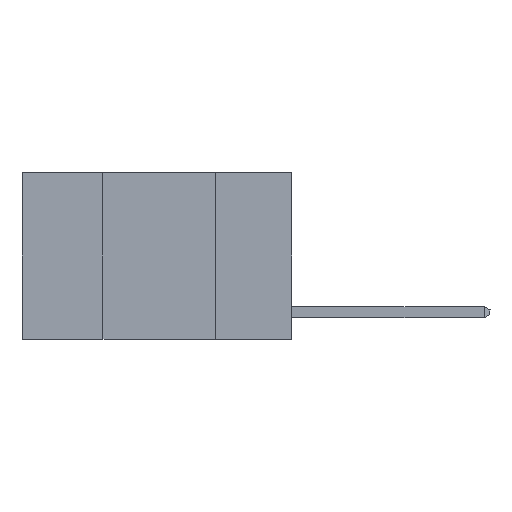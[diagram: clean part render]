
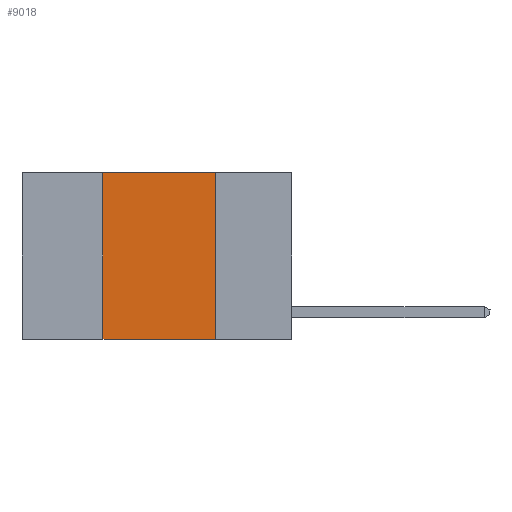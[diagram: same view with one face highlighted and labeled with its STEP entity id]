
A CAD part, left-side view. The second image highlights one B-rep face of the part: STEP entity #9018.
In plain terms, the highlighted planar face has unit normal (-1, 0, 0).
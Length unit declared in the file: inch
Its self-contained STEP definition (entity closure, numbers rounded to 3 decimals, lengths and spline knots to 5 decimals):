
#171 = VECTOR ( 'NONE', #7071, 39.37008 ) ;
#3466 = VERTEX_POINT ( 'NONE', #5015 ) ;
#3481 = CARTESIAN_POINT ( 'NONE',  ( 0., 0.6, -0.37 ) ) ;
#3925 = VECTOR ( 'NONE', #14369, 39.37008 ) ;
#5015 = CARTESIAN_POINT ( 'NONE',  ( 0., 0.17, 0. ) ) ;
#5437 = CARTESIAN_POINT ( 'NONE',  ( 0., 0.42, -0.37 ) ) ;
#6284 = DIRECTION ( 'NONE',  ( 1., 0., 0. ) ) ;
#7063 = VECTOR ( 'NONE', #12515, 39.37008 ) ;
#7071 = DIRECTION ( 'NONE',  ( 0., 0., 1. ) ) ;
#7338 = LINE ( 'NONE', #7885, #14939 ) ;
#7378 = ORIENTED_EDGE ( 'NONE', *, *, #17467, .F. ) ;
#7527 = AXIS2_PLACEMENT_3D ( 'NONE', #15374, #6284, #16900 ) ;
#7839 = VERTEX_POINT ( 'NONE', #8434 ) ;
#7885 = CARTESIAN_POINT ( 'NONE',  ( 0., 0.17, 0. ) ) ;
#7903 = EDGE_CURVE ( 'NONE', #10601, #18689, #12953, .T. ) ;
#8434 = CARTESIAN_POINT ( 'NONE',  ( 0., 0.17, -0.37 ) ) ;
#9018 = ADVANCED_FACE ( 'NONE', ( #11711 ), #16834, .F. ) ;
#9217 = EDGE_CURVE ( 'NONE', #18689, #3466, #11939, .T. ) ;
#9403 = DIRECTION ( 'NONE',  ( 0., 0., -1. ) ) ;
#10601 = VERTEX_POINT ( 'NONE', #5437 ) ;
#11711 = FACE_OUTER_BOUND ( 'NONE', #13921, .T. ) ;
#11939 = LINE ( 'NONE', #15851, #3925 ) ;
#12515 = DIRECTION ( 'NONE',  ( 0., -1., 0. ) ) ;
#12953 = LINE ( 'NONE', #19242, #171 ) ;
#13100 = EDGE_CURVE ( 'NONE', #10601, #7839, #15621, .T. ) ;
#13921 = EDGE_LOOP ( 'NONE', ( #7378, #17489, #14425, #15009 ) ) ;
#14369 = DIRECTION ( 'NONE',  ( 0., -1., 0. ) ) ;
#14425 = ORIENTED_EDGE ( 'NONE', *, *, #7903, .F. ) ;
#14939 = VECTOR ( 'NONE', #9403, 39.37008 ) ;
#15009 = ORIENTED_EDGE ( 'NONE', *, *, #13100, .T. ) ;
#15374 = CARTESIAN_POINT ( 'NONE',  ( 0., 0.6, 0. ) ) ;
#15621 = LINE ( 'NONE', #3481, #7063 ) ;
#15851 = CARTESIAN_POINT ( 'NONE',  ( 0., 0.6, 0. ) ) ;
#16834 = PLANE ( 'NONE',  #7527 ) ;
#16900 = DIRECTION ( 'NONE',  ( 0., 0., -1. ) ) ;
#17467 = EDGE_CURVE ( 'NONE', #3466, #7839, #7338, .T. ) ;
#17489 = ORIENTED_EDGE ( 'NONE', *, *, #9217, .F. ) ;
#17578 = CARTESIAN_POINT ( 'NONE',  ( 0., 0.42, 0. ) ) ;
#18689 = VERTEX_POINT ( 'NONE', #17578 ) ;
#19242 = CARTESIAN_POINT ( 'NONE',  ( 0., 0.42, 0. ) ) ;
